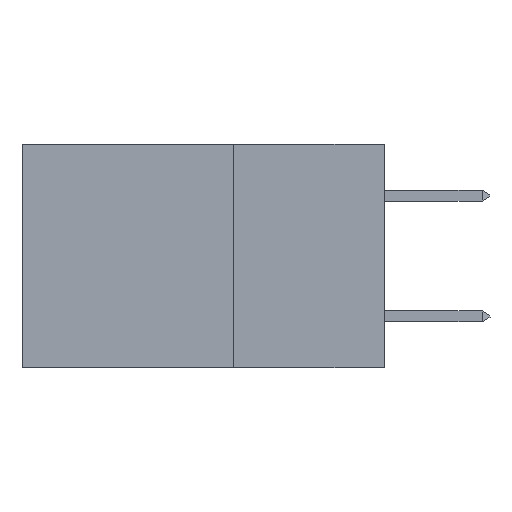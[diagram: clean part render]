
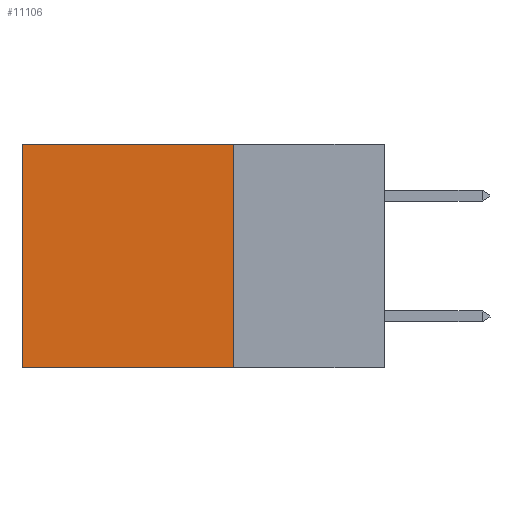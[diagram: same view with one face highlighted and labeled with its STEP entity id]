
A CAD part, left-side view. The second image highlights one B-rep face of the part: STEP entity #11106.
In plain terms, the highlighted planar face has unit normal (-1, 0, 0).
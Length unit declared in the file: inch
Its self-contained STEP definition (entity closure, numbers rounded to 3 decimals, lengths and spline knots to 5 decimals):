
#13 = CARTESIAN_POINT ( 'NONE',  ( 0.2875, 0.6, 0. ) ) ;
#994 = DIRECTION ( 'NONE',  ( 0., 0., -1. ) ) ;
#1233 = ORIENTED_EDGE ( 'NONE', *, *, #8695, .F. ) ;
#3066 = AXIS2_PLACEMENT_3D ( 'NONE', #17917, #10305, #994 ) ;
#3279 = VECTOR ( 'NONE', #15482, 39.37008 ) ;
#3459 = VECTOR ( 'NONE', #15488, 39.37008 ) ;
#4803 = VERTEX_POINT ( 'NONE', #16616 ) ;
#5522 = ORIENTED_EDGE ( 'NONE', *, *, #16781, .T. ) ;
#5685 = PLANE ( 'NONE',  #3066 ) ;
#6966 = EDGE_LOOP ( 'NONE', ( #5522, #9643, #1233, #12091 ) ) ;
#7028 = LINE ( 'NONE', #14775, #18769 ) ;
#7103 = DIRECTION ( 'NONE',  ( 0., 1., 0. ) ) ;
#7272 = VECTOR ( 'NONE', #16789, 39.37008 ) ;
#7961 = VERTEX_POINT ( 'NONE', #10616 ) ;
#7977 = EDGE_CURVE ( 'NONE', #7961, #9125, #19928, .T. ) ;
#8305 = CARTESIAN_POINT ( 'NONE',  ( 0.2875, 0.6, -0.37 ) ) ;
#8695 = EDGE_CURVE ( 'NONE', #7961, #4803, #16350, .T. ) ;
#9125 = VERTEX_POINT ( 'NONE', #10574 ) ;
#9134 = CARTESIAN_POINT ( 'NONE',  ( 0.2875, 0.25, 0. ) ) ;
#9643 = ORIENTED_EDGE ( 'NONE', *, *, #10248, .F. ) ;
#10248 = EDGE_CURVE ( 'NONE', #4803, #15697, #7028, .T. ) ;
#10305 = DIRECTION ( 'NONE',  ( 1., 0., 0. ) ) ;
#10574 = CARTESIAN_POINT ( 'NONE',  ( 0.2875, 0.6, 0. ) ) ;
#10616 = CARTESIAN_POINT ( 'NONE',  ( 0.2875, 0.25, 0. ) ) ;
#11106 = ADVANCED_FACE ( 'NONE', ( #19660 ), #5685, .F. ) ;
#11634 = LINE ( 'NONE', #13, #3459 ) ;
#12091 = ORIENTED_EDGE ( 'NONE', *, *, #7977, .T. ) ;
#12362 = CARTESIAN_POINT ( 'NONE',  ( 0.2875, 0.25, 0. ) ) ;
#14775 = CARTESIAN_POINT ( 'NONE',  ( 0.2875, 0.25, -0.37 ) ) ;
#15482 = DIRECTION ( 'NONE',  ( 0., 0., -1. ) ) ;
#15488 = DIRECTION ( 'NONE',  ( 0., 0., -1. ) ) ;
#15697 = VERTEX_POINT ( 'NONE', #8305 ) ;
#16350 = LINE ( 'NONE', #12362, #3279 ) ;
#16616 = CARTESIAN_POINT ( 'NONE',  ( 0.2875, 0.25, -0.37 ) ) ;
#16781 = EDGE_CURVE ( 'NONE', #9125, #15697, #11634, .T. ) ;
#16789 = DIRECTION ( 'NONE',  ( 0., 1., 0. ) ) ;
#17917 = CARTESIAN_POINT ( 'NONE',  ( 0.2875, 0.25, 0. ) ) ;
#18769 = VECTOR ( 'NONE', #7103, 39.37008 ) ;
#19660 = FACE_OUTER_BOUND ( 'NONE', #6966, .T. ) ;
#19928 = LINE ( 'NONE', #9134, #7272 ) ;
